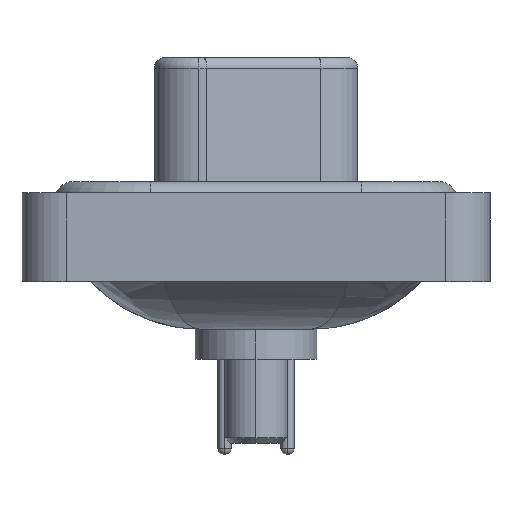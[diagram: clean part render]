
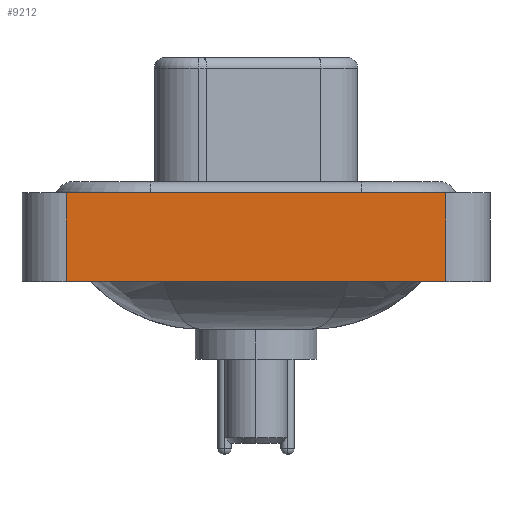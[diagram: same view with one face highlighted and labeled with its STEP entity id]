
A CAD part, left-side view. The second image highlights one B-rep face of the part: STEP entity #9212.
In plain terms, the highlighted planar face has unit normal (-1, 0, 0).
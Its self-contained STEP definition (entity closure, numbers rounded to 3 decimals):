
#68 = LINE ( 'NONE', #3848, #1343 ) ;
#545 = ORIENTED_EDGE ( 'NONE', *, *, #17025, .T. ) ;
#1343 = VECTOR ( 'NONE', #19594, 1000. ) ;
#2255 = CARTESIAN_POINT ( 'NONE',  ( -7.35, -8.55, -3.6 ) ) ;
#2435 = EDGE_CURVE ( 'NONE', #9061, #14322, #14299, .T. ) ;
#2673 = DIRECTION ( 'NONE',  ( 0., 0., 1. ) ) ;
#3103 = FACE_OUTER_BOUND ( 'NONE', #4390, .T. ) ;
#3145 = VERTEX_POINT ( 'NONE', #21318 ) ;
#3848 = CARTESIAN_POINT ( 'NONE',  ( -7.35, -8.55, -3.6 ) ) ;
#4390 = EDGE_LOOP ( 'NONE', ( #545, #8402, #10650, #11618 ) ) ;
#4446 = CARTESIAN_POINT ( 'NONE',  ( -7.35, 8.55, -3.6 ) ) ;
#5024 = VERTEX_POINT ( 'NONE', #7698 ) ;
#5147 = DIRECTION ( 'NONE',  ( 0., -1., 0. ) ) ;
#5585 = VECTOR ( 'NONE', #5147, 1000. ) ;
#7698 = CARTESIAN_POINT ( 'NONE',  ( -7.35, -8.55, 0.4 ) ) ;
#8402 = ORIENTED_EDGE ( 'NONE', *, *, #9887, .F. ) ;
#9061 = VERTEX_POINT ( 'NONE', #19907 ) ;
#9212 = ADVANCED_FACE ( 'NONE', ( #3103 ), #10513, .T. ) ;
#9574 = LINE ( 'NONE', #12973, #21345 ) ;
#9887 = EDGE_CURVE ( 'NONE', #3145, #5024, #9574, .T. ) ;
#10031 = CARTESIAN_POINT ( 'NONE',  ( -7.35, -8.55, -3.6 ) ) ;
#10513 = PLANE ( 'NONE',  #14373 ) ;
#10650 = ORIENTED_EDGE ( 'NONE', *, *, #16710, .F. ) ;
#10720 = VECTOR ( 'NONE', #2673, 1000. ) ;
#11618 = ORIENTED_EDGE ( 'NONE', *, *, #2435, .T. ) ;
#12973 = CARTESIAN_POINT ( 'NONE',  ( -7.35, -8.55, 0.4 ) ) ;
#14299 = LINE ( 'NONE', #14410, #5585 ) ;
#14322 = VERTEX_POINT ( 'NONE', #2255 ) ;
#14373 = AXIS2_PLACEMENT_3D ( 'NONE', #10031, #22750, #17410 ) ;
#14410 = CARTESIAN_POINT ( 'NONE',  ( -7.35, -8.55, -3.6 ) ) ;
#16710 = EDGE_CURVE ( 'NONE', #9061, #3145, #18563, .T. ) ;
#17025 = EDGE_CURVE ( 'NONE', #14322, #5024, #68, .T. ) ;
#17410 = DIRECTION ( 'NONE',  ( 0., 0., 1. ) ) ;
#18400 = DIRECTION ( 'NONE',  ( 0., -1., 0. ) ) ;
#18563 = LINE ( 'NONE', #4446, #10720 ) ;
#19594 = DIRECTION ( 'NONE',  ( 0., 0., 1. ) ) ;
#19907 = CARTESIAN_POINT ( 'NONE',  ( -7.35, 8.55, -3.6 ) ) ;
#21318 = CARTESIAN_POINT ( 'NONE',  ( -7.35, 8.55, 0.4 ) ) ;
#21345 = VECTOR ( 'NONE', #18400, 1000. ) ;
#22750 = DIRECTION ( 'NONE',  ( -1., 0., 0. ) ) ;
